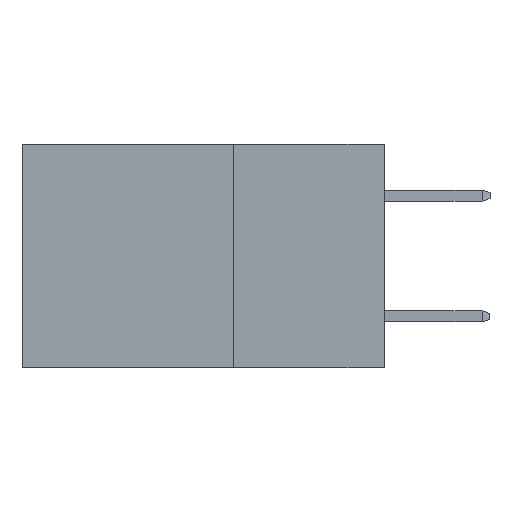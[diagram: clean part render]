
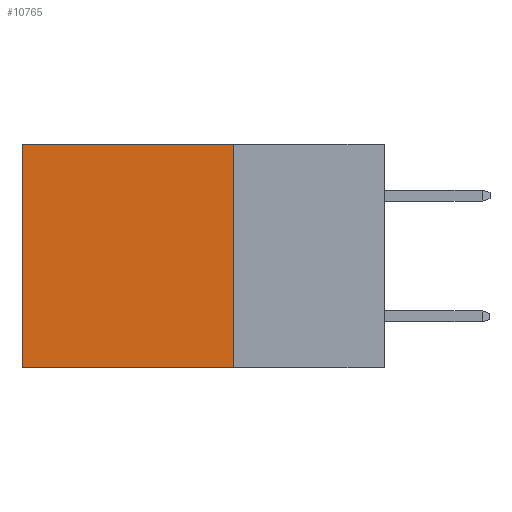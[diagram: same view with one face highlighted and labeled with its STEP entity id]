
A CAD part, left-side view. The second image highlights one B-rep face of the part: STEP entity #10765.
In plain terms, the highlighted planar face has unit normal (-1, 0, 0).
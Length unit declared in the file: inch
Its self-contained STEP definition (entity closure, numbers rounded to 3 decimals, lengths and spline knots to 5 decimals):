
#994 = LINE ( 'NONE', #7423, #8956 ) ;
#1331 = DIRECTION ( 'NONE',  ( 0., 0., -1. ) ) ;
#1433 = LINE ( 'NONE', #10734, #6252 ) ;
#1883 = FACE_OUTER_BOUND ( 'NONE', #1889, .T. ) ;
#1889 = EDGE_LOOP ( 'NONE', ( #6583, #11026, #12295, #8925 ) ) ;
#2161 = CARTESIAN_POINT ( 'NONE',  ( 0.298, 0.25, 0. ) ) ;
#2875 = CARTESIAN_POINT ( 'NONE',  ( 0.298, 0.25, 0. ) ) ;
#3100 = VERTEX_POINT ( 'NONE', #2161 ) ;
#3211 = EDGE_CURVE ( 'NONE', #3100, #10397, #994, .T. ) ;
#3920 = PLANE ( 'NONE',  #9804 ) ;
#4981 = DIRECTION ( 'NONE',  ( 1., 0., 0. ) ) ;
#5791 = LINE ( 'NONE', #8258, #6958 ) ;
#5809 = VERTEX_POINT ( 'NONE', #8854 ) ;
#6252 = VECTOR ( 'NONE', #12496, 39.37008 ) ;
#6275 = EDGE_CURVE ( 'NONE', #5809, #7054, #8171, .T. ) ;
#6583 = ORIENTED_EDGE ( 'NONE', *, *, #6275, .T. ) ;
#6958 = VECTOR ( 'NONE', #7339, 39.37008 ) ;
#7011 = EDGE_CURVE ( 'NONE', #10397, #7054, #1433, .T. ) ;
#7054 = VERTEX_POINT ( 'NONE', #9915 ) ;
#7339 = DIRECTION ( 'NONE',  ( 0., 1., 0. ) ) ;
#7423 = CARTESIAN_POINT ( 'NONE',  ( 0.298, 0.25, 0. ) ) ;
#7611 = VECTOR ( 'NONE', #8720, 39.37008 ) ;
#8171 = LINE ( 'NONE', #12225, #7611 ) ;
#8258 = CARTESIAN_POINT ( 'NONE',  ( 0.298, 0.25, 0. ) ) ;
#8720 = DIRECTION ( 'NONE',  ( 0., 0., -1. ) ) ;
#8854 = CARTESIAN_POINT ( 'NONE',  ( 0.298, 0.6, 0. ) ) ;
#8925 = ORIENTED_EDGE ( 'NONE', *, *, #9246, .T. ) ;
#8956 = VECTOR ( 'NONE', #1331, 39.37008 ) ;
#9240 = CARTESIAN_POINT ( 'NONE',  ( 0.298, 0.25, -0.37 ) ) ;
#9246 = EDGE_CURVE ( 'NONE', #3100, #5809, #5791, .T. ) ;
#9804 = AXIS2_PLACEMENT_3D ( 'NONE', #2875, #4981, #11385 ) ;
#9915 = CARTESIAN_POINT ( 'NONE',  ( 0.298, 0.6, -0.37 ) ) ;
#10397 = VERTEX_POINT ( 'NONE', #9240 ) ;
#10734 = CARTESIAN_POINT ( 'NONE',  ( 0.298, 0.25, -0.37 ) ) ;
#10765 = ADVANCED_FACE ( 'NONE', ( #1883 ), #3920, .F. ) ;
#11026 = ORIENTED_EDGE ( 'NONE', *, *, #7011, .F. ) ;
#11385 = DIRECTION ( 'NONE',  ( 0., 0., -1. ) ) ;
#12225 = CARTESIAN_POINT ( 'NONE',  ( 0.298, 0.6, 0. ) ) ;
#12295 = ORIENTED_EDGE ( 'NONE', *, *, #3211, .F. ) ;
#12496 = DIRECTION ( 'NONE',  ( 0., 1., 0. ) ) ;
